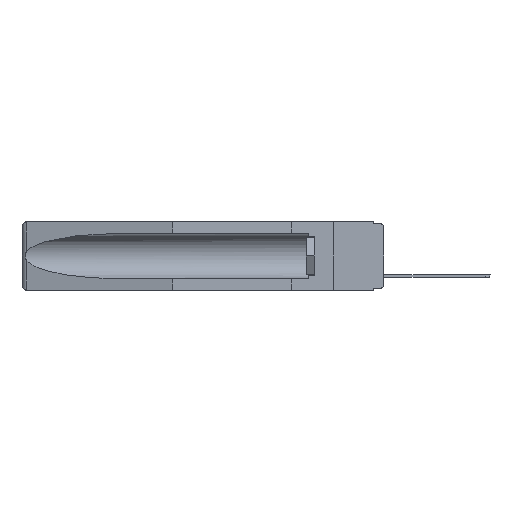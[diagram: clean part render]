
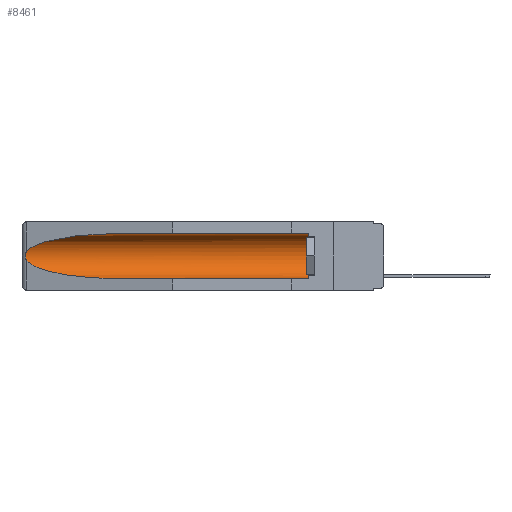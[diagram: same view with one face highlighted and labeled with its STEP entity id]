
A CAD part, left-side view. The second image highlights one B-rep face of the part: STEP entity #8461.
In plain terms, the highlighted cylindrical face has radius 2.857 mm (diameter 5.715 mm), a partial arc.
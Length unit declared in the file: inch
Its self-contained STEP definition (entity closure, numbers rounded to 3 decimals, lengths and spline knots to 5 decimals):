
#233 = EDGE_CURVE ( 'NONE', #3466, #17510, #12255, .T. ) ;
#1755 = CARTESIAN_POINT ( 'NONE',  ( 0.26597, 1.5296, -0.19026 ) ) ;
#2273 = DIRECTION ( 'NONE',  ( 0., 0., 1. ) ) ;
#2367 = CARTESIAN_POINT ( 'NONE',  ( 0.26537, 1.52718, -0.19328 ) ) ;
#2991 = EDGE_CURVE ( 'NONE', #4594, #19379, #9778, .T. ) ;
#3248 = CARTESIAN_POINT ( 'NONE',  ( 0.155, 0.126, -0.059 ) ) ;
#3466 = VERTEX_POINT ( 'NONE', #3248 ) ;
#4454 = AXIS2_PLACEMENT_3D ( 'NONE', #14487, #12976, #12836 ) ;
#4594 = VERTEX_POINT ( 'NONE', #20673 ) ;
#5023 = CARTESIAN_POINT ( 'NONE',  ( 0.155, -0.30754, -0.284 ) ) ;
#5110 = EDGE_CURVE ( 'NONE', #17510, #4594, #15148, .T. ) ;
#5432 = CARTESIAN_POINT ( 'NONE',  ( 0.155, 1.07973, -0.059 ) ) ;
#5868 = EDGE_LOOP ( 'NONE', ( #11270, #17149, #16230, #18163, #20983, #12788 ) ) ;
#5988 = VERTEX_POINT ( 'NONE', #6944 ) ;
#6182 = EDGE_CURVE ( 'NONE', #13227, #3466, #6613, .T. ) ;
#6340 = CARTESIAN_POINT ( 'NONE',  ( 0.26537, 1.52718, -0.19328 ) ) ;
#6613 = CIRCLE ( 'NONE', #9274, 0.1125 ) ;
#6871 = CARTESIAN_POINT ( 'NONE',  ( 0.2675, 1.53308, -0.17534 ) ) ;
#6934 = CARTESIAN_POINT ( 'NONE',  ( 0.155, -0.30754, -0.059 ) ) ;
#6945 = CARTESIAN_POINT ( 'NONE',  ( 0.2673, 1.5327, -0.16383 ) ) ;
#6944 = CARTESIAN_POINT ( 'NONE',  ( 0.155, 1.07973, -0.284 ) ) ;
#7011 = CARTESIAN_POINT ( 'NONE',  ( 0.26537, 1.52718, -0.14972 ) ) ;
#7085 = CARTESIAN_POINT ( 'NONE',  ( 0.2673, 1.53269, -0.17917 ) ) ;
#7143 = VECTOR ( 'NONE', #17098, 39.37008 ) ;
#7463 = CARTESIAN_POINT ( 'NONE',  ( 0.155, 0.126, -0.1715 ) ) ;
#8121 = VECTOR ( 'NONE', #19153, 39.37008 ) ;
#8461 = ADVANCED_FACE ( 'NONE', ( #16740 ), #13773, .F. ) ;
#8504 = CARTESIAN_POINT ( 'NONE',  ( 0.26537, 1.52718, -0.14972 ) ) ;
#8519 = EDGE_CURVE ( 'NONE', #13227, #5988, #21865, .T. ) ;
#8728 = CARTESIAN_POINT ( 'NONE',  ( 0.26654, 1.53092, -0.15636 ) ) ;
#8806 = CARTESIAN_POINT ( 'NONE',  ( 0.25451, 1.48313, -0.09465 ) ) ;
#9274 = AXIS2_PLACEMENT_3D ( 'NONE', #7463, #17931, #2273 ) ;
#9778 = B_SPLINE_CURVE_WITH_KNOTS ( 'NONE', 3,
 ( #8504, #15600, #8728, #6945, #18976, #6871, #7085, #19120, #1755, #20791 ),
 .UNSPECIFIED., .F., .F.,
 ( 4, 2, 2, 2, 4 ),
 ( 0., 0.00029, 0.00058, 0.00087, 0.00117 ),
 .UNSPECIFIED. ) ;
#10842 = CARTESIAN_POINT ( 'NONE',  ( 0.21114, 1.30732, -0.284 ) ) ;
#10922 = CARTESIAN_POINT ( 'NONE',  ( 0.155, 1.07973, -0.284 ) ) ;
#11270 = ORIENTED_EDGE ( 'NONE', *, *, #5110, .T. ) ;
#12255 = LINE ( 'NONE', #6934, #7143 ) ;
#12788 = ORIENTED_EDGE ( 'NONE', *, *, #233, .T. ) ;
#12836 = DIRECTION ( 'NONE',  ( 0., 0., 1. ) ) ;
#12976 = DIRECTION ( 'NONE',  ( 0., 1., 0. ) ) ;
#13227 = VERTEX_POINT ( 'NONE', #19665 ) ;
#13773 = CYLINDRICAL_SURFACE ( 'NONE', #4454, 0.1125 ) ;
#13779 = CARTESIAN_POINT ( 'NONE',  ( 0.21114, 1.30732, -0.059 ) ) ;
#14487 = CARTESIAN_POINT ( 'NONE',  ( 0.155, -0.30754, -0.1715 ) ) ;
#14905 = CARTESIAN_POINT ( 'NONE',  ( 0.155, 1.07973, -0.059 ) ) ;
#15148 =( BOUNDED_CURVE ( )  B_SPLINE_CURVE ( 3, ( #5432, #13779, #8806, #7011 ),
 .UNSPECIFIED., .F., .F. ) 
 B_SPLINE_CURVE_WITH_KNOTS ( ( 4, 4 ),
 ( 4.71239, 6.08839 ),
 .UNSPECIFIED. ) 
 CURVE ( )  GEOMETRIC_REPRESENTATION_ITEM ( )  RATIONAL_B_SPLINE_CURVE ( ( 1., 0.848, 0.848, 1. ) ) 
 REPRESENTATION_ITEM ( '' )  );
#15600 = CARTESIAN_POINT ( 'NONE',  ( 0.26597, 1.52961, -0.15275 ) ) ;
#16230 = ORIENTED_EDGE ( 'NONE', *, *, #20710, .T. ) ;
#16740 = FACE_OUTER_BOUND ( 'NONE', #5868, .T. ) ;
#17098 = DIRECTION ( 'NONE',  ( 0., 1., 0. ) ) ;
#17149 = ORIENTED_EDGE ( 'NONE', *, *, #2991, .T. ) ;
#17510 = VERTEX_POINT ( 'NONE', #14905 ) ;
#17931 = DIRECTION ( 'NONE',  ( 0., -1., 0. ) ) ;
#18163 = ORIENTED_EDGE ( 'NONE', *, *, #8519, .F. ) ;
#18211 =( BOUNDED_CURVE ( )  B_SPLINE_CURVE ( 3, ( #2367, #19441, #10842, #10922 ),
 .UNSPECIFIED., .F., .F. ) 
 B_SPLINE_CURVE_WITH_KNOTS ( ( 4, 4 ),
 ( 0.1948, 1.5708 ),
 .UNSPECIFIED. ) 
 CURVE ( )  GEOMETRIC_REPRESENTATION_ITEM ( )  RATIONAL_B_SPLINE_CURVE ( ( 1., 0.848, 0.848, 1. ) ) 
 REPRESENTATION_ITEM ( '' )  );
#18976 = CARTESIAN_POINT ( 'NONE',  ( 0.2675, 1.53308, -0.16763 ) ) ;
#19120 = CARTESIAN_POINT ( 'NONE',  ( 0.26655, 1.53094, -0.18657 ) ) ;
#19153 = DIRECTION ( 'NONE',  ( 0., 1., 0. ) ) ;
#19379 = VERTEX_POINT ( 'NONE', #6340 ) ;
#19441 = CARTESIAN_POINT ( 'NONE',  ( 0.25451, 1.48313, -0.24835 ) ) ;
#19665 = CARTESIAN_POINT ( 'NONE',  ( 0.155, 0.126, -0.284 ) ) ;
#20673 = CARTESIAN_POINT ( 'NONE',  ( 0.26537, 1.52718, -0.14972 ) ) ;
#20710 = EDGE_CURVE ( 'NONE', #19379, #5988, #18211, .T. ) ;
#20791 = CARTESIAN_POINT ( 'NONE',  ( 0.26537, 1.52718, -0.19328 ) ) ;
#20983 = ORIENTED_EDGE ( 'NONE', *, *, #6182, .T. ) ;
#21865 = LINE ( 'NONE', #5023, #8121 ) ;
